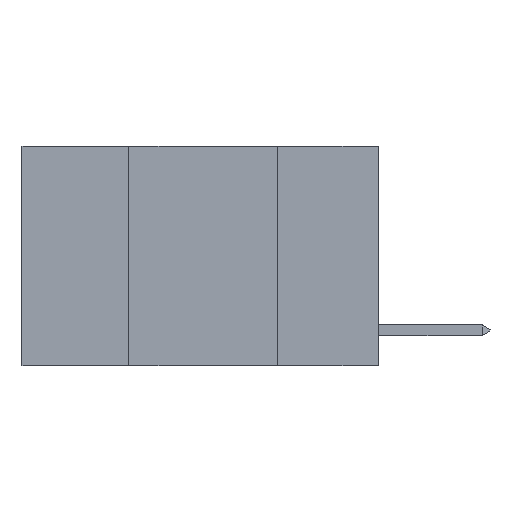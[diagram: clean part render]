
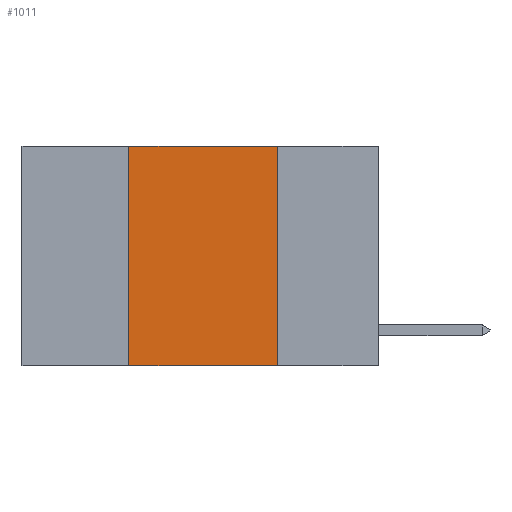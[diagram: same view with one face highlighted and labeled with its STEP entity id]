
A CAD part, left-side view. The second image highlights one B-rep face of the part: STEP entity #1011.
In plain terms, the highlighted planar face has unit normal (-1, 0, 0).
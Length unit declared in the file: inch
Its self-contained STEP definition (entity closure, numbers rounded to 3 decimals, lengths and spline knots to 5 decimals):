
#372 = ORIENTED_EDGE ( 'NONE', *, *, #14861, .F. ) ;
#1011 = ADVANCED_FACE ( 'NONE', ( #14671 ), #20232, .F. ) ;
#1885 = ORIENTED_EDGE ( 'NONE', *, *, #15709, .F. ) ;
#2446 = CARTESIAN_POINT ( 'NONE',  ( 0., 0.42, -0.37 ) ) ;
#2512 = CARTESIAN_POINT ( 'NONE',  ( 0., 0.17, 0. ) ) ;
#3103 = EDGE_LOOP ( 'NONE', ( #372, #1885, #8075, #8003 ) ) ;
#4086 = CARTESIAN_POINT ( 'NONE',  ( 0., 0.6, 0. ) ) ;
#4291 = LINE ( 'NONE', #2512, #13746 ) ;
#4862 = DIRECTION ( 'NONE',  ( 0., 0., -1. ) ) ;
#5167 = VECTOR ( 'NONE', #20870, 39.37008 ) ;
#5980 = CARTESIAN_POINT ( 'NONE',  ( 0., 0.17, 0. ) ) ;
#6215 = VECTOR ( 'NONE', #11434, 39.37008 ) ;
#6419 = VECTOR ( 'NONE', #11650, 39.37008 ) ;
#7127 = AXIS2_PLACEMENT_3D ( 'NONE', #4086, #11458, #15369 ) ;
#8003 = ORIENTED_EDGE ( 'NONE', *, *, #22391, .T. ) ;
#8075 = ORIENTED_EDGE ( 'NONE', *, *, #14555, .F. ) ;
#9472 = VERTEX_POINT ( 'NONE', #5980 ) ;
#10595 = CARTESIAN_POINT ( 'NONE',  ( 0., 0.17, -0.37 ) ) ;
#11434 = DIRECTION ( 'NONE',  ( 0., 0., 1. ) ) ;
#11458 = DIRECTION ( 'NONE',  ( 1., 0., 0. ) ) ;
#11524 = LINE ( 'NONE', #17194, #5167 ) ;
#11650 = DIRECTION ( 'NONE',  ( 0., -1., 0. ) ) ;
#13746 = VECTOR ( 'NONE', #4862, 39.37008 ) ;
#14346 = VERTEX_POINT ( 'NONE', #17911 ) ;
#14555 = EDGE_CURVE ( 'NONE', #21493, #14346, #18765, .T. ) ;
#14671 = FACE_OUTER_BOUND ( 'NONE', #3103, .T. ) ;
#14861 = EDGE_CURVE ( 'NONE', #9472, #20883, #4291, .T. ) ;
#15369 = DIRECTION ( 'NONE',  ( 0., 0., -1. ) ) ;
#15709 = EDGE_CURVE ( 'NONE', #14346, #9472, #18532, .T. ) ;
#17194 = CARTESIAN_POINT ( 'NONE',  ( 0., 0.6, -0.37 ) ) ;
#17911 = CARTESIAN_POINT ( 'NONE',  ( 0., 0.42, 0. ) ) ;
#18532 = LINE ( 'NONE', #20530, #6419 ) ;
#18765 = LINE ( 'NONE', #18875, #6215 ) ;
#18875 = CARTESIAN_POINT ( 'NONE',  ( 0., 0.42, 0. ) ) ;
#20232 = PLANE ( 'NONE',  #7127 ) ;
#20530 = CARTESIAN_POINT ( 'NONE',  ( 0., 0.6, 0. ) ) ;
#20870 = DIRECTION ( 'NONE',  ( 0., -1., 0. ) ) ;
#20883 = VERTEX_POINT ( 'NONE', #10595 ) ;
#21493 = VERTEX_POINT ( 'NONE', #2446 ) ;
#22391 = EDGE_CURVE ( 'NONE', #21493, #20883, #11524, .T. ) ;
